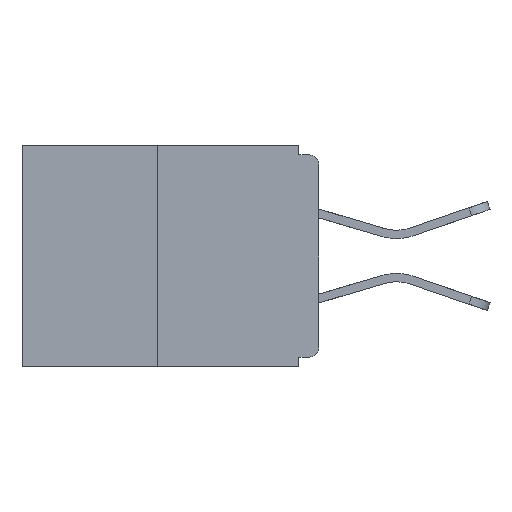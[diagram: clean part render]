
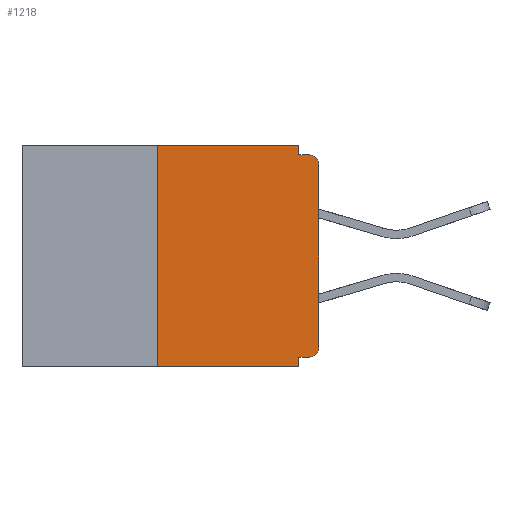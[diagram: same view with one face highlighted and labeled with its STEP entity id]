
A CAD part, left-side view. The second image highlights one B-rep face of the part: STEP entity #1218.
In plain terms, the highlighted planar face has unit normal (-1, 0, 0).
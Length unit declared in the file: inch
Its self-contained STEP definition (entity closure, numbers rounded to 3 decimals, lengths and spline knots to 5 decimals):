
#183 = EDGE_CURVE ( 'NONE', #9699, #7238, #14191, .T. ) ;
#740 = CARTESIAN_POINT ( 'NONE',  ( 0., 0.015, -0.015 ) ) ;
#878 = VECTOR ( 'NONE', #13336, 39.37008 ) ;
#1218 = ADVANCED_FACE ( 'NONE', ( #20840 ), #4390, .F. ) ;
#2394 = ORIENTED_EDGE ( 'NONE', *, *, #4120, .F. ) ;
#2852 = EDGE_CURVE ( 'NONE', #5849, #20694, #8713, .T. ) ;
#3260 = DIRECTION ( 'NONE',  ( 0., -1., 0. ) ) ;
#4043 = VECTOR ( 'NONE', #13965, 39.37008 ) ;
#4120 = EDGE_CURVE ( 'NONE', #19818, #8351, #20737, .T. ) ;
#4390 = PLANE ( 'NONE',  #20885 ) ;
#4413 = CARTESIAN_POINT ( 'NONE',  ( 0., 0.25, 0. ) ) ;
#4488 = DIRECTION ( 'NONE',  ( 0., 0., 1. ) ) ;
#5065 = LINE ( 'NONE', #10796, #4043 ) ;
#5218 = DIRECTION ( 'NONE',  ( 0., 1., 0. ) ) ;
#5229 = CARTESIAN_POINT ( 'NONE',  ( 0., 0.25, 0. ) ) ;
#5608 = DIRECTION ( 'NONE',  ( 0., -1., 0. ) ) ;
#5825 = VECTOR ( 'NONE', #3260, 39.37008 ) ;
#5849 = VERTEX_POINT ( 'NONE', #6063 ) ;
#5870 = DIRECTION ( 'NONE',  ( 0., 0., -1. ) ) ;
#5987 = ORIENTED_EDGE ( 'NONE', *, *, #183, .T. ) ;
#6063 = CARTESIAN_POINT ( 'NONE',  ( 0., 0.015, -0.328 ) ) ;
#6301 = DIRECTION ( 'NONE',  ( 0., 0., -1. ) ) ;
#6797 = CARTESIAN_POINT ( 'NONE',  ( 0., 0., 0. ) ) ;
#7238 = VERTEX_POINT ( 'NONE', #740 ) ;
#7339 = DIRECTION ( 'NONE',  ( 0., -1., 0. ) ) ;
#7482 = CARTESIAN_POINT ( 'NONE',  ( 0., 0.46, 0. ) ) ;
#7485 = CARTESIAN_POINT ( 'NONE',  ( 0., 0.015, -0.313 ) ) ;
#7661 = ORIENTED_EDGE ( 'NONE', *, *, #17366, .T. ) ;
#7855 = CARTESIAN_POINT ( 'NONE',  ( 0., 0.031, -0.343 ) ) ;
#8351 = VERTEX_POINT ( 'NONE', #14159 ) ;
#8547 = CARTESIAN_POINT ( 'NONE',  ( 0., 0., -0.328 ) ) ;
#8713 = LINE ( 'NONE', #8547, #14359 ) ;
#8776 = ORIENTED_EDGE ( 'NONE', *, *, #2852, .F. ) ;
#8780 = VECTOR ( 'NONE', #4488, 39.37008 ) ;
#8875 = CARTESIAN_POINT ( 'NONE',  ( 0., 0.031, -0.328 ) ) ;
#8921 = ORIENTED_EDGE ( 'NONE', *, *, #10313, .F. ) ;
#9159 = VERTEX_POINT ( 'NONE', #17917 ) ;
#9162 = LINE ( 'NONE', #7482, #10205 ) ;
#9216 = DIRECTION ( 'NONE',  ( 0., 0., -1. ) ) ;
#9488 = DIRECTION ( 'NONE',  ( -1., 0., 0. ) ) ;
#9621 = LINE ( 'NONE', #6797, #878 ) ;
#9699 = VERTEX_POINT ( 'NONE', #21327 ) ;
#9846 = ORIENTED_EDGE ( 'NONE', *, *, #12429, .T. ) ;
#9989 = EDGE_CURVE ( 'NONE', #9159, #10868, #13562, .T. ) ;
#10085 = VERTEX_POINT ( 'NONE', #15117 ) ;
#10205 = VECTOR ( 'NONE', #7339, 39.37008 ) ;
#10313 = EDGE_CURVE ( 'NONE', #8351, #7238, #15115, .T. ) ;
#10796 = CARTESIAN_POINT ( 'NONE',  ( 0., 0.031, -0.343 ) ) ;
#10868 = VERTEX_POINT ( 'NONE', #7855 ) ;
#10899 = CIRCLE ( 'NONE', #18532, 0.015 ) ;
#11200 = CARTESIAN_POINT ( 'NONE',  ( 0., 0.015, -0.03 ) ) ;
#12393 = EDGE_LOOP ( 'NONE', ( #21079, #17250, #18795, #17171, #8776, #9846, #7661, #5987, #8921, #2394 ) ) ;
#12429 = EDGE_CURVE ( 'NONE', #5849, #10085, #10899, .T. ) ;
#12710 = DIRECTION ( 'NONE',  ( 0., 0., -1. ) ) ;
#13336 = DIRECTION ( 'NONE',  ( 0., 0., 1. ) ) ;
#13562 = LINE ( 'NONE', #15482, #20787 ) ;
#13851 = CARTESIAN_POINT ( 'NONE',  ( 0., 0.031, 0. ) ) ;
#13965 = DIRECTION ( 'NONE',  ( 0., 0., -1. ) ) ;
#14034 = DIRECTION ( 'NONE',  ( 1., 0., 0. ) ) ;
#14159 = CARTESIAN_POINT ( 'NONE',  ( 0., 0.031, -0.015 ) ) ;
#14191 = CIRCLE ( 'NONE', #19931, 0.015 ) ;
#14256 = VERTEX_POINT ( 'NONE', #5229 ) ;
#14293 = VECTOR ( 'NONE', #6301, 39.37008 ) ;
#14359 = VECTOR ( 'NONE', #5218, 39.37008 ) ;
#15115 = LINE ( 'NONE', #18091, #5825 ) ;
#15117 = CARTESIAN_POINT ( 'NONE',  ( 0., 0., -0.313 ) ) ;
#15482 = CARTESIAN_POINT ( 'NONE',  ( 0., 0.46, -0.343 ) ) ;
#15633 = CARTESIAN_POINT ( 'NONE',  ( 0., 0.46, 0. ) ) ;
#15751 = DIRECTION ( 'NONE',  ( -1., 0., 0. ) ) ;
#16230 = CARTESIAN_POINT ( 'NONE',  ( 0., 0.031, 0. ) ) ;
#17171 = ORIENTED_EDGE ( 'NONE', *, *, #20618, .F. ) ;
#17250 = ORIENTED_EDGE ( 'NONE', *, *, #18506, .F. ) ;
#17366 = EDGE_CURVE ( 'NONE', #10085, #9699, #9621, .T. ) ;
#17917 = CARTESIAN_POINT ( 'NONE',  ( 0., 0.25, -0.343 ) ) ;
#18091 = CARTESIAN_POINT ( 'NONE',  ( 0., 0., -0.015 ) ) ;
#18506 = EDGE_CURVE ( 'NONE', #9159, #14256, #19353, .T. ) ;
#18532 = AXIS2_PLACEMENT_3D ( 'NONE', #7485, #15751, #5870 ) ;
#18795 = ORIENTED_EDGE ( 'NONE', *, *, #9989, .T. ) ;
#19353 = LINE ( 'NONE', #4413, #8780 ) ;
#19818 = VERTEX_POINT ( 'NONE', #13851 ) ;
#19931 = AXIS2_PLACEMENT_3D ( 'NONE', #11200, #9488, #12710 ) ;
#19976 = EDGE_CURVE ( 'NONE', #14256, #19818, #9162, .T. ) ;
#20618 = EDGE_CURVE ( 'NONE', #20694, #10868, #5065, .T. ) ;
#20694 = VERTEX_POINT ( 'NONE', #8875 ) ;
#20737 = LINE ( 'NONE', #16230, #14293 ) ;
#20787 = VECTOR ( 'NONE', #5608, 39.37008 ) ;
#20840 = FACE_OUTER_BOUND ( 'NONE', #12393, .T. ) ;
#20885 = AXIS2_PLACEMENT_3D ( 'NONE', #15633, #14034, #9216 ) ;
#21079 = ORIENTED_EDGE ( 'NONE', *, *, #19976, .F. ) ;
#21327 = CARTESIAN_POINT ( 'NONE',  ( 0., 0., -0.03 ) ) ;
